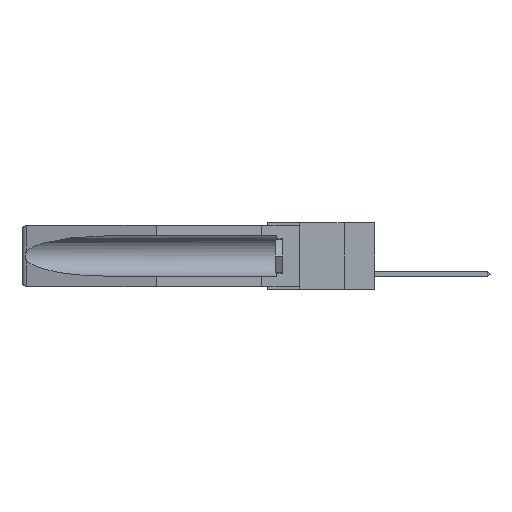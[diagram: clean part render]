
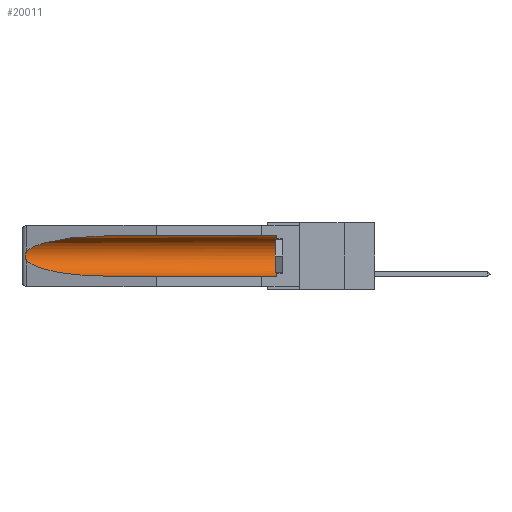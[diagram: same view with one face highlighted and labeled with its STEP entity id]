
A CAD part, left-side view. The second image highlights one B-rep face of the part: STEP entity #20011.
In plain terms, the highlighted cylindrical face has radius 2.857 mm (diameter 5.715 mm), a partial arc.
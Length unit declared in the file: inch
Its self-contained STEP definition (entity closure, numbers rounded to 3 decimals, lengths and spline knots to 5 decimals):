
#771 = CARTESIAN_POINT ( 'NONE',  ( 0.155, 0.126, -0.059 ) ) ;
#1185 = DIRECTION ( 'NONE',  ( 0., 1., 0. ) ) ;
#1209 = CARTESIAN_POINT ( 'NONE',  ( 0.26537, 1.52718, -0.19328 ) ) ;
#1307 = CARTESIAN_POINT ( 'NONE',  ( 0.2675, 1.53308, -0.16763 ) ) ;
#1399 = CARTESIAN_POINT ( 'NONE',  ( 0.2673, 1.5327, -0.16383 ) ) ;
#1510 = CARTESIAN_POINT ( 'NONE',  ( 0.21114, 1.30732, -0.284 ) ) ;
#1524 = CARTESIAN_POINT ( 'NONE',  ( 0.26655, 1.53094, -0.18657 ) ) ;
#2318 = VERTEX_POINT ( 'NONE', #3707 ) ;
#2741 = EDGE_LOOP ( 'NONE', ( #21292, #20489, #20907, #12898, #20265, #19920 ) ) ;
#3456 = CARTESIAN_POINT ( 'NONE',  ( 0.26537, 1.52718, -0.19328 ) ) ;
#3707 = CARTESIAN_POINT ( 'NONE',  ( 0.26537, 1.52718, -0.14972 ) ) ;
#4454 = CARTESIAN_POINT ( 'NONE',  ( 0.155, 1.07973, -0.059 ) ) ;
#4989 = LINE ( 'NONE', #13416, #19170 ) ;
#5249 = VECTOR ( 'NONE', #15707, 39.37008 ) ;
#5430 = VERTEX_POINT ( 'NONE', #7213 ) ;
#5929 = CARTESIAN_POINT ( 'NONE',  ( 0.155, -0.30754, -0.1715 ) ) ;
#6634 = B_SPLINE_CURVE_WITH_KNOTS ( 'NONE', 3,
 ( #15511, #12872, #15624, #1399, #1307, #20226, #22411, #1524, #25085, #1209 ),
 .UNSPECIFIED., .F., .F.,
 ( 4, 2, 2, 2, 4 ),
 ( 0., 0.00029, 0.00058, 0.00087, 0.00117 ),
 .UNSPECIFIED. ) ;
#6782 = DIRECTION ( 'NONE',  ( 0., 0., 1. ) ) ;
#7213 = CARTESIAN_POINT ( 'NONE',  ( 0.155, 1.07973, -0.284 ) ) ;
#8095 = CARTESIAN_POINT ( 'NONE',  ( 0.26537, 1.52718, -0.19328 ) ) ;
#8678 = VERTEX_POINT ( 'NONE', #771 ) ;
#8701 = VERTEX_POINT ( 'NONE', #8095 ) ;
#9985 = AXIS2_PLACEMENT_3D ( 'NONE', #5929, #1185, #27223 ) ;
#10971 = CARTESIAN_POINT ( 'NONE',  ( 0.155, 0.126, -0.284 ) ) ;
#12147 = EDGE_CURVE ( 'NONE', #27481, #2318, #19610, .T. ) ;
#12872 = CARTESIAN_POINT ( 'NONE',  ( 0.26597, 1.52961, -0.15275 ) ) ;
#12898 = ORIENTED_EDGE ( 'NONE', *, *, #20039, .F. ) ;
#13416 = CARTESIAN_POINT ( 'NONE',  ( 0.155, -0.30754, -0.059 ) ) ;
#13597 = CARTESIAN_POINT ( 'NONE',  ( 0.25451, 1.48313, -0.09465 ) ) ;
#13687 = EDGE_CURVE ( 'NONE', #8678, #27481, #4989, .T. ) ;
#14136 = VERTEX_POINT ( 'NONE', #10971 ) ;
#14531 = EDGE_CURVE ( 'NONE', #14136, #8678, #24337, .T. ) ;
#15511 = CARTESIAN_POINT ( 'NONE',  ( 0.26537, 1.52718, -0.14972 ) ) ;
#15624 = CARTESIAN_POINT ( 'NONE',  ( 0.26654, 1.53092, -0.15636 ) ) ;
#15707 = DIRECTION ( 'NONE',  ( 0., 1., 0. ) ) ;
#16055 = CARTESIAN_POINT ( 'NONE',  ( 0.155, 0.126, -0.1715 ) ) ;
#17904 = FACE_OUTER_BOUND ( 'NONE', #2741, .T. ) ;
#19170 = VECTOR ( 'NONE', #30361, 39.37008 ) ;
#19610 =( BOUNDED_CURVE ( )  B_SPLINE_CURVE ( 3, ( #4454, #20814, #13597, #23199 ),
 .UNSPECIFIED., .F., .F. ) 
 B_SPLINE_CURVE_WITH_KNOTS ( ( 4, 4 ),
 ( 4.71239, 6.08839 ),
 .UNSPECIFIED. ) 
 CURVE ( )  GEOMETRIC_REPRESENTATION_ITEM ( )  RATIONAL_B_SPLINE_CURVE ( ( 1., 0.848, 0.848, 1. ) ) 
 REPRESENTATION_ITEM ( '' )  );
#19920 = ORIENTED_EDGE ( 'NONE', *, *, #13687, .T. ) ;
#20011 = ADVANCED_FACE ( 'NONE', ( #17904 ), #21658, .F. ) ;
#20039 = EDGE_CURVE ( 'NONE', #14136, #5430, #26464, .T. ) ;
#20226 = CARTESIAN_POINT ( 'NONE',  ( 0.2675, 1.53308, -0.17534 ) ) ;
#20265 = ORIENTED_EDGE ( 'NONE', *, *, #14531, .T. ) ;
#20489 = ORIENTED_EDGE ( 'NONE', *, *, #24080, .T. ) ;
#20814 = CARTESIAN_POINT ( 'NONE',  ( 0.21114, 1.30732, -0.059 ) ) ;
#20907 = ORIENTED_EDGE ( 'NONE', *, *, #27121, .T. ) ;
#21292 = ORIENTED_EDGE ( 'NONE', *, *, #12147, .T. ) ;
#21658 = CYLINDRICAL_SURFACE ( 'NONE', #9985, 0.1125 ) ;
#22411 = CARTESIAN_POINT ( 'NONE',  ( 0.2673, 1.53269, -0.17917 ) ) ;
#22485 = CARTESIAN_POINT ( 'NONE',  ( 0.155, 1.07973, -0.284 ) ) ;
#23182 = CARTESIAN_POINT ( 'NONE',  ( 0.155, 1.07973, -0.059 ) ) ;
#23199 = CARTESIAN_POINT ( 'NONE',  ( 0.26537, 1.52718, -0.14972 ) ) ;
#23227 = DIRECTION ( 'NONE',  ( 0., -1., 0. ) ) ;
#24080 = EDGE_CURVE ( 'NONE', #2318, #8701, #6634, .T. ) ;
#24337 = CIRCLE ( 'NONE', #25252, 0.1125 ) ;
#24976 = CARTESIAN_POINT ( 'NONE',  ( 0.25451, 1.48313, -0.24835 ) ) ;
#25085 = CARTESIAN_POINT ( 'NONE',  ( 0.26597, 1.5296, -0.19026 ) ) ;
#25252 = AXIS2_PLACEMENT_3D ( 'NONE', #16055, #23227, #6782 ) ;
#26464 = LINE ( 'NONE', #30023, #5249 ) ;
#27121 = EDGE_CURVE ( 'NONE', #8701, #5430, #27363, .T. ) ;
#27223 = DIRECTION ( 'NONE',  ( 0., 0., 1. ) ) ;
#27363 =( BOUNDED_CURVE ( )  B_SPLINE_CURVE ( 3, ( #3456, #24976, #1510, #22485 ),
 .UNSPECIFIED., .F., .T. ) 
 B_SPLINE_CURVE_WITH_KNOTS ( ( 4, 4 ),
 ( 0.1948, 1.5708 ),
 .UNSPECIFIED. ) 
 CURVE ( )  GEOMETRIC_REPRESENTATION_ITEM ( )  RATIONAL_B_SPLINE_CURVE ( ( 1., 0.848, 0.848, 1. ) ) 
 REPRESENTATION_ITEM ( '' )  );
#27481 = VERTEX_POINT ( 'NONE', #23182 ) ;
#30023 = CARTESIAN_POINT ( 'NONE',  ( 0.155, -0.30754, -0.284 ) ) ;
#30361 = DIRECTION ( 'NONE',  ( 0., 1., 0. ) ) ;
